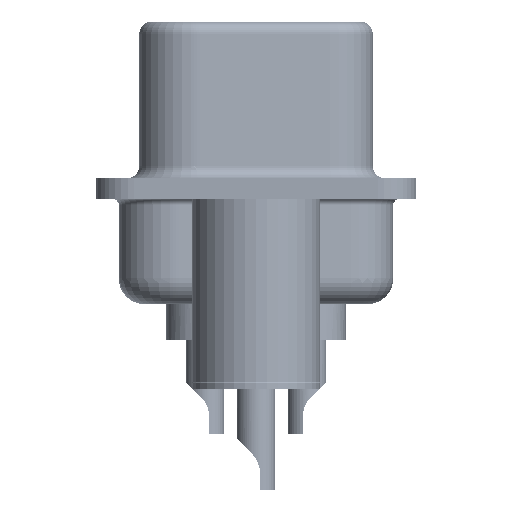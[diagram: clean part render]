
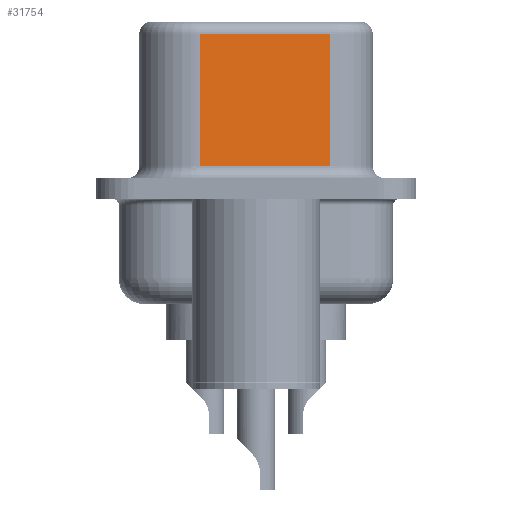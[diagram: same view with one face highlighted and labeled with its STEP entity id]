
A CAD part, left-side view. The second image highlights one B-rep face of the part: STEP entity #31754.
In plain terms, the highlighted planar face has unit normal (-0.985, -0.174, 0).
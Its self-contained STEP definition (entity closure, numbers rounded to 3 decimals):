
#744 = VECTOR ( 'NONE', #20193, 1000. ) ;
#2207 = CARTESIAN_POINT ( 'NONE',  ( 4.58, -2.897, 0.9 ) ) ;
#3719 = VECTOR ( 'NONE', #27376, 1000. ) ;
#4419 = CARTESIAN_POINT ( 'NONE',  ( 3.68, 2.203, 6.02 ) ) ;
#4653 = VERTEX_POINT ( 'NONE', #8319 ) ;
#5001 = EDGE_CURVE ( 'NONE', #18137, #31037, #30995, .T. ) ;
#5369 = VECTOR ( 'NONE', #10817, 1000. ) ;
#6480 = DIRECTION ( 'NONE',  ( -0.174, 0.985, 0. ) ) ;
#6703 = AXIS2_PLACEMENT_3D ( 'NONE', #31997, #21770, #6480 ) ;
#7924 = DIRECTION ( 'NONE',  ( -0.174, 0.985, 0. ) ) ;
#8319 = CARTESIAN_POINT ( 'NONE',  ( 4.58, -2.897, 0.9 ) ) ;
#8380 = FACE_OUTER_BOUND ( 'NONE', #9629, .T. ) ;
#8458 = ORIENTED_EDGE ( 'NONE', *, *, #14723, .F. ) ;
#9040 = PLANE ( 'NONE',  #6703 ) ;
#9629 = EDGE_LOOP ( 'NONE', ( #8458, #18377, #23701, #12172 ) ) ;
#9844 = CARTESIAN_POINT ( 'NONE',  ( 3.68, 2.203, 0.9 ) ) ;
#10817 = DIRECTION ( 'NONE',  ( 0., 0., -1. ) ) ;
#12172 = ORIENTED_EDGE ( 'NONE', *, *, #21475, .T. ) ;
#14723 = EDGE_CURVE ( 'NONE', #18137, #4653, #24135, .T. ) ;
#15526 = CARTESIAN_POINT ( 'NONE',  ( 4.58, -2.897, 6.02 ) ) ;
#17347 = CARTESIAN_POINT ( 'NONE',  ( 4.58, -2.897, 6.02 ) ) ;
#18137 = VERTEX_POINT ( 'NONE', #17347 ) ;
#18377 = ORIENTED_EDGE ( 'NONE', *, *, #5001, .T. ) ;
#20193 = DIRECTION ( 'NONE',  ( 0.174, -0.985, 0. ) ) ;
#20468 = LINE ( 'NONE', #2207, #744 ) ;
#21475 = EDGE_CURVE ( 'NONE', #33211, #4653, #20468, .T. ) ;
#21770 = DIRECTION ( 'NONE',  ( 0.985, 0.174, 0. ) ) ;
#23701 = ORIENTED_EDGE ( 'NONE', *, *, #25788, .T. ) ;
#24130 = VECTOR ( 'NONE', #7924, 1000. ) ;
#24135 = LINE ( 'NONE', #27698, #3719 ) ;
#25788 = EDGE_CURVE ( 'NONE', #31037, #33211, #31820, .T. ) ;
#27376 = DIRECTION ( 'NONE',  ( 0., 0., -1. ) ) ;
#27698 = CARTESIAN_POINT ( 'NONE',  ( 4.58, -2.897, 6.52 ) ) ;
#28592 = CARTESIAN_POINT ( 'NONE',  ( 3.68, 2.203, 6.52 ) ) ;
#30995 = LINE ( 'NONE', #15526, #24130 ) ;
#31037 = VERTEX_POINT ( 'NONE', #4419 ) ;
#31754 = ADVANCED_FACE ( 'NONE', ( #8380 ), #9040, .F. ) ;
#31820 = LINE ( 'NONE', #28592, #5369 ) ;
#31997 = CARTESIAN_POINT ( 'NONE',  ( 4.58, -2.897, 6.52 ) ) ;
#33211 = VERTEX_POINT ( 'NONE', #9844 ) ;
